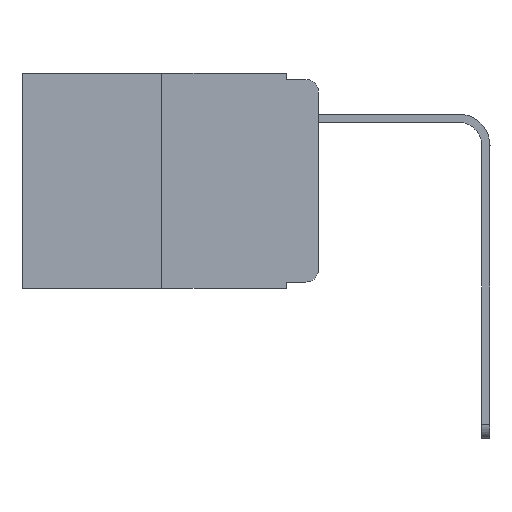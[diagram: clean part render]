
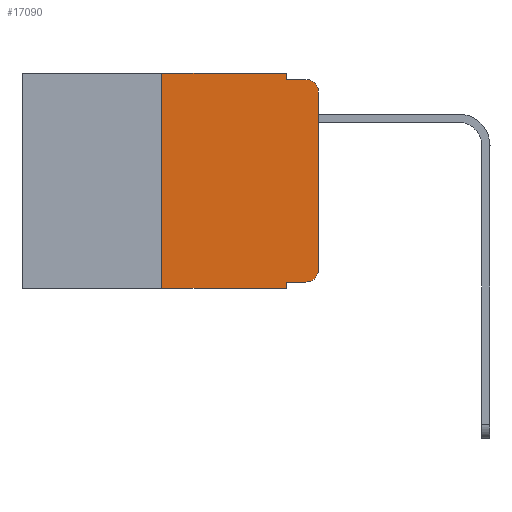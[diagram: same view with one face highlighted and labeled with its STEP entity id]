
A CAD part, left-side view. The second image highlights one B-rep face of the part: STEP entity #17090.
In plain terms, the highlighted planar face has unit normal (-1, 0, 0).
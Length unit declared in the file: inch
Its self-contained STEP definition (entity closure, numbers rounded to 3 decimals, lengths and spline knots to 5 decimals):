
#16 = CARTESIAN_POINT ( 'NONE',  ( 0., 0.051, -0.333 ) ) ;
#263 = CARTESIAN_POINT ( 'NONE',  ( 0., 0., -0.313 ) ) ;
#380 = ORIENTED_EDGE ( 'NONE', *, *, #9526, .F. ) ;
#408 = CARTESIAN_POINT ( 'NONE',  ( 0., 0.051, 0. ) ) ;
#608 = DIRECTION ( 'NONE',  ( -1., 0., 0. ) ) ;
#644 = ORIENTED_EDGE ( 'NONE', *, *, #5688, .T. ) ;
#673 = CARTESIAN_POINT ( 'NONE',  ( 0., 0.051, -0.01 ) ) ;
#1049 = LINE ( 'NONE', #14672, #8319 ) ;
#1350 = ORIENTED_EDGE ( 'NONE', *, *, #15647, .T. ) ;
#1624 = ORIENTED_EDGE ( 'NONE', *, *, #17110, .F. ) ;
#1913 = DIRECTION ( 'NONE',  ( 0., 0., -1. ) ) ;
#2116 = LINE ( 'NONE', #9372, #14465 ) ;
#2225 = VERTEX_POINT ( 'NONE', #4019 ) ;
#2803 = ORIENTED_EDGE ( 'NONE', *, *, #14230, .T. ) ;
#3453 = CARTESIAN_POINT ( 'NONE',  ( 0., 0.051, 0. ) ) ;
#3629 = CIRCLE ( 'NONE', #10397, 0.02 ) ;
#3688 = DIRECTION ( 'NONE',  ( -1., 0., 0. ) ) ;
#3712 = LINE ( 'NONE', #4911, #9006 ) ;
#3808 = DIRECTION ( 'NONE',  ( 0., 0., -1. ) ) ;
#3884 = DIRECTION ( 'NONE',  ( 0., -1., 0. ) ) ;
#4019 = CARTESIAN_POINT ( 'NONE',  ( 0., 0.02, -0.333 ) ) ;
#4029 = CIRCLE ( 'NONE', #4756, 0.02 ) ;
#4420 = CARTESIAN_POINT ( 'NONE',  ( 0., 0.473, -0.343 ) ) ;
#4513 = CARTESIAN_POINT ( 'NONE',  ( 0., 0.473, 0. ) ) ;
#4756 = AXIS2_PLACEMENT_3D ( 'NONE', #9415, #3688, #3808 ) ;
#4816 = LINE ( 'NONE', #16116, #12543 ) ;
#4911 = CARTESIAN_POINT ( 'NONE',  ( 0., 0.051, -0.333 ) ) ;
#4963 = DIRECTION ( 'NONE',  ( 0., 0., -1. ) ) ;
#5045 = ORIENTED_EDGE ( 'NONE', *, *, #15268, .F. ) ;
#5383 = PLANE ( 'NONE',  #15854 ) ;
#5688 = EDGE_CURVE ( 'NONE', #11819, #2225, #3712, .T. ) ;
#5698 = ORIENTED_EDGE ( 'NONE', *, *, #5801, .F. ) ;
#5801 = EDGE_CURVE ( 'NONE', #11819, #7388, #4816, .T. ) ;
#5977 = DIRECTION ( 'NONE',  ( 0., -1., 0. ) ) ;
#6013 = CARTESIAN_POINT ( 'NONE',  ( 0., 0.25, -0.343 ) ) ;
#6149 = CARTESIAN_POINT ( 'NONE',  ( 0., 0.02, -0.01 ) ) ;
#6264 = LINE ( 'NONE', #13776, #17042 ) ;
#7343 = VECTOR ( 'NONE', #11831, 39.37008 ) ;
#7388 = VERTEX_POINT ( 'NONE', #11015 ) ;
#7454 = VERTEX_POINT ( 'NONE', #6149 ) ;
#7902 = CARTESIAN_POINT ( 'NONE',  ( 0., 0.25, 0. ) ) ;
#8201 = CARTESIAN_POINT ( 'NONE',  ( 0., 0.473, 0. ) ) ;
#8319 = VECTOR ( 'NONE', #17517, 39.37008 ) ;
#8323 = VERTEX_POINT ( 'NONE', #7902 ) ;
#8580 = ORIENTED_EDGE ( 'NONE', *, *, #17547, .T. ) ;
#8995 = CARTESIAN_POINT ( 'NONE',  ( 0., 0.02, -0.03 ) ) ;
#9006 = VECTOR ( 'NONE', #10568, 39.37008 ) ;
#9372 = CARTESIAN_POINT ( 'NONE',  ( 0., 0.051, -0.01 ) ) ;
#9415 = CARTESIAN_POINT ( 'NONE',  ( 0., 0.02, -0.313 ) ) ;
#9526 = EDGE_CURVE ( 'NONE', #8323, #16180, #13282, .T. ) ;
#9583 = VERTEX_POINT ( 'NONE', #263 ) ;
#10214 = EDGE_LOOP ( 'NONE', ( #16862, #1350, #5045, #11552, #380, #1624, #2803, #5698, #644, #8580 ) ) ;
#10397 = AXIS2_PLACEMENT_3D ( 'NONE', #8995, #608, #1913 ) ;
#10568 = DIRECTION ( 'NONE',  ( 0., -1., 0. ) ) ;
#11015 = CARTESIAN_POINT ( 'NONE',  ( 0., 0.051, -0.343 ) ) ;
#11036 = DIRECTION ( 'NONE',  ( 0., 0., -1. ) ) ;
#11457 = VERTEX_POINT ( 'NONE', #14454 ) ;
#11552 = ORIENTED_EDGE ( 'NONE', *, *, #17403, .F. ) ;
#11819 = VERTEX_POINT ( 'NONE', #16 ) ;
#11831 = DIRECTION ( 'NONE',  ( 0., 0., -1. ) ) ;
#12543 = VECTOR ( 'NONE', #4963, 39.37008 ) ;
#13039 = DIRECTION ( 'NONE',  ( 0., -1., 0. ) ) ;
#13282 = LINE ( 'NONE', #4513, #16590 ) ;
#13406 = VECTOR ( 'NONE', #5977, 39.37008 ) ;
#13771 = FACE_OUTER_BOUND ( 'NONE', #10214, .T. ) ;
#13776 = CARTESIAN_POINT ( 'NONE',  ( 0., 0.25, 0. ) ) ;
#14076 = DIRECTION ( 'NONE',  ( 0., 0., 1. ) ) ;
#14230 = EDGE_CURVE ( 'NONE', #14971, #7388, #17545, .T. ) ;
#14454 = CARTESIAN_POINT ( 'NONE',  ( 0., 0., -0.03 ) ) ;
#14465 = VECTOR ( 'NONE', #3884, 39.37008 ) ;
#14467 = EDGE_CURVE ( 'NONE', #9583, #11457, #1049, .T. ) ;
#14672 = CARTESIAN_POINT ( 'NONE',  ( 0., 0., 0. ) ) ;
#14971 = VERTEX_POINT ( 'NONE', #6013 ) ;
#15072 = LINE ( 'NONE', #3453, #7343 ) ;
#15268 = EDGE_CURVE ( 'NONE', #15787, #7454, #2116, .T. ) ;
#15647 = EDGE_CURVE ( 'NONE', #11457, #7454, #3629, .T. ) ;
#15787 = VERTEX_POINT ( 'NONE', #673 ) ;
#15854 = AXIS2_PLACEMENT_3D ( 'NONE', #8201, #18020, #11036 ) ;
#16116 = CARTESIAN_POINT ( 'NONE',  ( 0., 0.051, 0. ) ) ;
#16180 = VERTEX_POINT ( 'NONE', #408 ) ;
#16590 = VECTOR ( 'NONE', #13039, 39.37008 ) ;
#16862 = ORIENTED_EDGE ( 'NONE', *, *, #14467, .T. ) ;
#17042 = VECTOR ( 'NONE', #14076, 39.37008 ) ;
#17090 = ADVANCED_FACE ( 'NONE', ( #13771 ), #5383, .F. ) ;
#17110 = EDGE_CURVE ( 'NONE', #14971, #8323, #6264, .T. ) ;
#17403 = EDGE_CURVE ( 'NONE', #16180, #15787, #15072, .T. ) ;
#17517 = DIRECTION ( 'NONE',  ( 0., 0., 1. ) ) ;
#17545 = LINE ( 'NONE', #4420, #13406 ) ;
#17547 = EDGE_CURVE ( 'NONE', #2225, #9583, #4029, .T. ) ;
#18020 = DIRECTION ( 'NONE',  ( 1., 0., 0. ) ) ;
